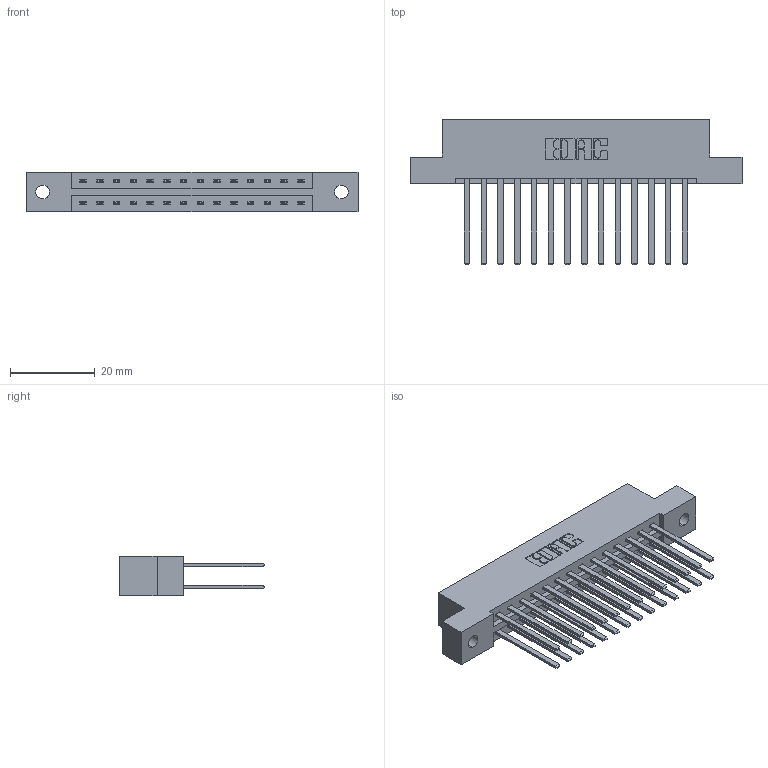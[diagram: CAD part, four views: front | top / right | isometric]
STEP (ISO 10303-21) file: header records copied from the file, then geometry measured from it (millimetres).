
FILE_DESCRIPTION (( 'STEP AP203' ), '1' );
FILE_NAME ('387-028-544-202.STEP', '2019-10-16T22:26:09', ( '' ), ( '' ), 'SwSTEP 2.0', 'SolidWorks 2016', '' );
FILE_SCHEMA (( 'CONFIG_CONTROL_DESIGN' ));
Length unit declared in the file: inch
Products named in the file (3): 337 Part_Flush Mounting Lugs - 0.128 Dia; 387-028-544-202; 345-292-001_345-293-144
Assembly tree (29 placements, depth 2):
  387-028-544-202
    337 Part_Flush Mounting Lugs - 0.128 Dia
    345-292-001_345-293-144  x28
Bounding box: 78.49 x 34.3 x 9.4 mm (x, y, z)
Volume: 8254.6 mm3; surface area: 10069.4 mm2
Topology: 29 solids, 29 shells, 1458 faces, 4315 edges, 2838 vertices
Faces by surface type: plane 1022, cylinder 436
Entity records: 14295 total; most frequent: CARTESIAN_POINT 2430, ORIENTED_EDGE 2366, DIRECTION 2115, EDGE_CURVE 1183, VECTOR 1059, LINE 1059, VERTEX_POINT 786, AXIS2_PLACEMENT_3D 528
